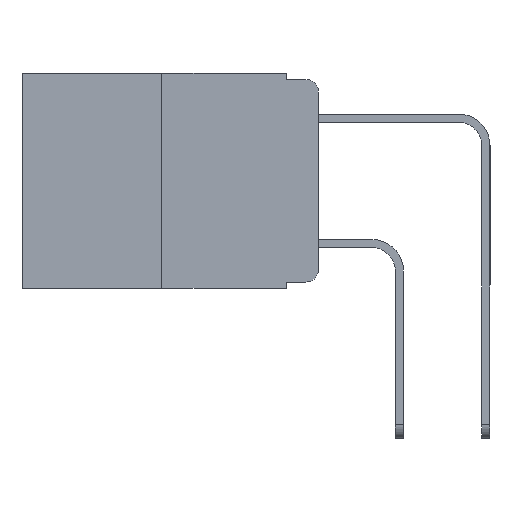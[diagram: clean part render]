
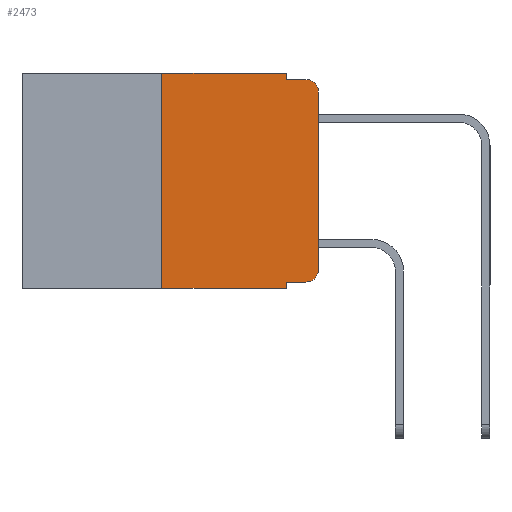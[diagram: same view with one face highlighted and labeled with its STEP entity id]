
A CAD part, left-side view. The second image highlights one B-rep face of the part: STEP entity #2473.
In plain terms, the highlighted planar face has unit normal (-1, 0, 0).
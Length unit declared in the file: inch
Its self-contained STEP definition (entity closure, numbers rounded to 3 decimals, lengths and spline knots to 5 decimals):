
#407 = ORIENTED_EDGE ( 'NONE', *, *, #11998, .F. ) ;
#433 = DIRECTION ( 'NONE',  ( 0., -1., 0. ) ) ;
#589 = EDGE_CURVE ( 'NONE', #2095, #3004, #12297, .T. ) ;
#829 = EDGE_CURVE ( 'NONE', #8386, #10167, #11704, .T. ) ;
#877 = VECTOR ( 'NONE', #15911, 39.37008 ) ;
#1522 = CARTESIAN_POINT ( 'NONE',  ( 0., 0.051, 0. ) ) ;
#2021 = CARTESIAN_POINT ( 'NONE',  ( 0., 0.051, -0.333 ) ) ;
#2095 = VERTEX_POINT ( 'NONE', #10767 ) ;
#2431 = DIRECTION ( 'NONE',  ( 1., 0., 0. ) ) ;
#2473 = ADVANCED_FACE ( 'NONE', ( #15857 ), #17174, .F. ) ;
#2734 = VECTOR ( 'NONE', #8502, 39.37008 ) ;
#2817 = EDGE_CURVE ( 'NONE', #15624, #3004, #8382, .T. ) ;
#3004 = VERTEX_POINT ( 'NONE', #8699 ) ;
#3310 = CARTESIAN_POINT ( 'NONE',  ( 0., 0.473, 0. ) ) ;
#3535 = DIRECTION ( 'NONE',  ( 0., -1., 0. ) ) ;
#3889 = DIRECTION ( 'NONE',  ( -1., 0., 0. ) ) ;
#4190 = DIRECTION ( 'NONE',  ( -1., 0., 0. ) ) ;
#4310 = DIRECTION ( 'NONE',  ( 0., -1., 0. ) ) ;
#4490 = ORIENTED_EDGE ( 'NONE', *, *, #589, .T. ) ;
#5023 = CARTESIAN_POINT ( 'NONE',  ( 0., 0., -0.313 ) ) ;
#5093 = LINE ( 'NONE', #5359, #877 ) ;
#5359 = CARTESIAN_POINT ( 'NONE',  ( 0., 0., 0. ) ) ;
#5616 = DIRECTION ( 'NONE',  ( 0., 0., 1. ) ) ;
#5831 = VECTOR ( 'NONE', #10626, 39.37008 ) ;
#5987 = CARTESIAN_POINT ( 'NONE',  ( 0., 0.02, -0.313 ) ) ;
#6077 = VERTEX_POINT ( 'NONE', #9544 ) ;
#6509 = EDGE_CURVE ( 'NONE', #15624, #8386, #7862, .T. ) ;
#6534 = EDGE_CURVE ( 'NONE', #7742, #11687, #17287, .T. ) ;
#6915 = AXIS2_PLACEMENT_3D ( 'NONE', #5987, #4190, #9818 ) ;
#7133 = CARTESIAN_POINT ( 'NONE',  ( 0., 0.051, 0. ) ) ;
#7249 = CARTESIAN_POINT ( 'NONE',  ( 0., 0.051, -0.01 ) ) ;
#7557 = ORIENTED_EDGE ( 'NONE', *, *, #14525, .T. ) ;
#7586 = DIRECTION ( 'NONE',  ( 0., 0., -1. ) ) ;
#7596 = CARTESIAN_POINT ( 'NONE',  ( 0., 0., -0.03 ) ) ;
#7742 = VERTEX_POINT ( 'NONE', #8522 ) ;
#7862 = LINE ( 'NONE', #16572, #11031 ) ;
#8096 = AXIS2_PLACEMENT_3D ( 'NONE', #10822, #2431, #7586 ) ;
#8378 = EDGE_CURVE ( 'NONE', #11687, #15666, #16435, .T. ) ;
#8382 = LINE ( 'NONE', #15089, #10731 ) ;
#8386 = VERTEX_POINT ( 'NONE', #13804 ) ;
#8502 = DIRECTION ( 'NONE',  ( 0., 0., -1. ) ) ;
#8522 = CARTESIAN_POINT ( 'NONE',  ( 0., 0.25, 0. ) ) ;
#8699 = CARTESIAN_POINT ( 'NONE',  ( 0., 0.051, -0.343 ) ) ;
#9114 = CIRCLE ( 'NONE', #13640, 0.02 ) ;
#9317 = EDGE_CURVE ( 'NONE', #2095, #7742, #12517, .T. ) ;
#9480 = ORIENTED_EDGE ( 'NONE', *, *, #829, .T. ) ;
#9544 = CARTESIAN_POINT ( 'NONE',  ( 0., 0.02, -0.01 ) ) ;
#9818 = DIRECTION ( 'NONE',  ( 0., 0., -1. ) ) ;
#10167 = VERTEX_POINT ( 'NONE', #5023 ) ;
#10547 = ORIENTED_EDGE ( 'NONE', *, *, #9317, .F. ) ;
#10616 = VECTOR ( 'NONE', #4310, 39.37008 ) ;
#10626 = DIRECTION ( 'NONE',  ( 0., -1., 0. ) ) ;
#10731 = VECTOR ( 'NONE', #15874, 39.37008 ) ;
#10767 = CARTESIAN_POINT ( 'NONE',  ( 0., 0.25, -0.343 ) ) ;
#10822 = CARTESIAN_POINT ( 'NONE',  ( 0., 0.473, 0. ) ) ;
#10957 = VERTEX_POINT ( 'NONE', #7596 ) ;
#11031 = VECTOR ( 'NONE', #433, 39.37008 ) ;
#11114 = EDGE_CURVE ( 'NONE', #10957, #6077, #9114, .T. ) ;
#11153 = ORIENTED_EDGE ( 'NONE', *, *, #11114, .T. ) ;
#11687 = VERTEX_POINT ( 'NONE', #1522 ) ;
#11704 = CIRCLE ( 'NONE', #6915, 0.02 ) ;
#11910 = VECTOR ( 'NONE', #3535, 39.37008 ) ;
#11998 = EDGE_CURVE ( 'NONE', #15666, #6077, #13033, .T. ) ;
#12042 = CARTESIAN_POINT ( 'NONE',  ( 0., 0.02, -0.03 ) ) ;
#12297 = LINE ( 'NONE', #15976, #11910 ) ;
#12370 = ORIENTED_EDGE ( 'NONE', *, *, #6534, .F. ) ;
#12395 = CARTESIAN_POINT ( 'NONE',  ( 0., 0.25, 0. ) ) ;
#12517 = LINE ( 'NONE', #12395, #15424 ) ;
#12603 = ORIENTED_EDGE ( 'NONE', *, *, #6509, .T. ) ;
#13033 = LINE ( 'NONE', #14437, #5831 ) ;
#13341 = DIRECTION ( 'NONE',  ( 0., 0., -1. ) ) ;
#13640 = AXIS2_PLACEMENT_3D ( 'NONE', #12042, #3889, #13341 ) ;
#13804 = CARTESIAN_POINT ( 'NONE',  ( 0., 0.02, -0.333 ) ) ;
#14437 = CARTESIAN_POINT ( 'NONE',  ( 0., 0.051, -0.01 ) ) ;
#14525 = EDGE_CURVE ( 'NONE', #10167, #10957, #5093, .T. ) ;
#15089 = CARTESIAN_POINT ( 'NONE',  ( 0., 0.051, 0. ) ) ;
#15298 = ORIENTED_EDGE ( 'NONE', *, *, #8378, .F. ) ;
#15424 = VECTOR ( 'NONE', #5616, 39.37008 ) ;
#15501 = ORIENTED_EDGE ( 'NONE', *, *, #2817, .F. ) ;
#15624 = VERTEX_POINT ( 'NONE', #2021 ) ;
#15666 = VERTEX_POINT ( 'NONE', #7249 ) ;
#15857 = FACE_OUTER_BOUND ( 'NONE', #16231, .T. ) ;
#15874 = DIRECTION ( 'NONE',  ( 0., 0., -1. ) ) ;
#15911 = DIRECTION ( 'NONE',  ( 0., 0., 1. ) ) ;
#15976 = CARTESIAN_POINT ( 'NONE',  ( 0., 0.473, -0.343 ) ) ;
#16231 = EDGE_LOOP ( 'NONE', ( #7557, #11153, #407, #15298, #12370, #10547, #4490, #15501, #12603, #9480 ) ) ;
#16435 = LINE ( 'NONE', #7133, #2734 ) ;
#16572 = CARTESIAN_POINT ( 'NONE',  ( 0., 0.051, -0.333 ) ) ;
#17174 = PLANE ( 'NONE',  #8096 ) ;
#17287 = LINE ( 'NONE', #3310, #10616 ) ;
